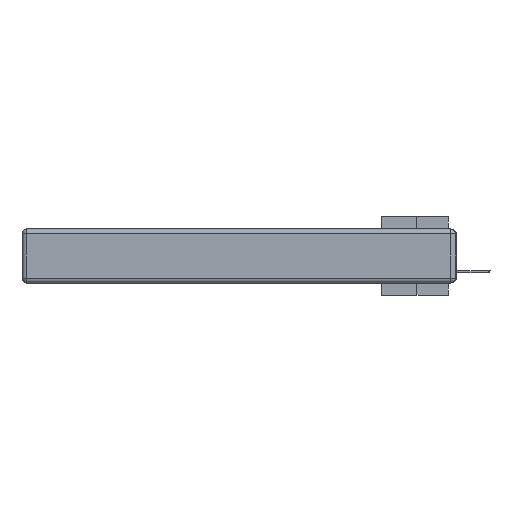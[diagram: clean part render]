
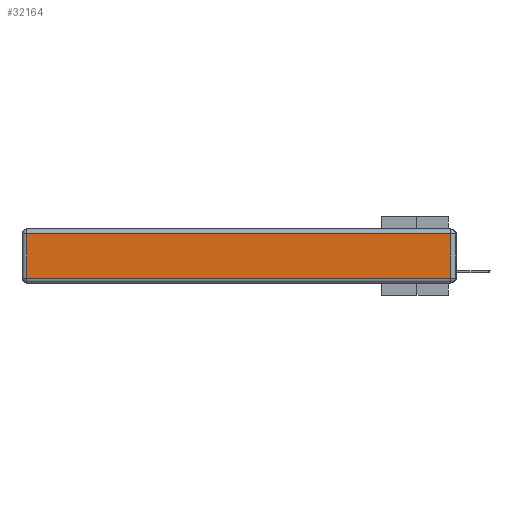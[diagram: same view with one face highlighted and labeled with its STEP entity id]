
A CAD part, left-side view. The second image highlights one B-rep face of the part: STEP entity #32164.
In plain terms, the highlighted planar face has unit normal (-1, 0, 0).
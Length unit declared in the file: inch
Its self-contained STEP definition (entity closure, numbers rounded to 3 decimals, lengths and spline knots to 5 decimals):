
#1705 = ORIENTED_EDGE ( 'NONE', *, *, #19413, .T. ) ;
#3553 = VECTOR ( 'NONE', #9380, 39.37008 ) ;
#4396 = VERTEX_POINT ( 'NONE', #17899 ) ;
#5908 = EDGE_LOOP ( 'NONE', ( #1705, #12740, #26076, #20247 ) ) ;
#6373 = CARTESIAN_POINT ( 'NONE',  ( 0., 0., -0.343 ) ) ;
#6792 = VERTEX_POINT ( 'NONE', #34179 ) ;
#7459 = DIRECTION ( 'NONE',  ( 0., -1., 0. ) ) ;
#8401 = VECTOR ( 'NONE', #7459, 39.37008 ) ;
#8530 = VECTOR ( 'NONE', #11083, 39.37008 ) ;
#9243 = DIRECTION ( 'NONE',  ( -1., 0., 0. ) ) ;
#9380 = DIRECTION ( 'NONE',  ( 0., 1., 0. ) ) ;
#9867 = LINE ( 'NONE', #18057, #3553 ) ;
#10703 = FACE_OUTER_BOUND ( 'NONE', #5908, .T. ) ;
#10829 = CARTESIAN_POINT ( 'NONE',  ( 0., 2.72, -0.343 ) ) ;
#11083 = DIRECTION ( 'NONE',  ( 0., 0., -1. ) ) ;
#11346 = VERTEX_POINT ( 'NONE', #35079 ) ;
#12740 = ORIENTED_EDGE ( 'NONE', *, *, #19407, .T. ) ;
#15490 = DIRECTION ( 'NONE',  ( 0., 0., 1. ) ) ;
#16065 = EDGE_CURVE ( 'NONE', #26657, #6792, #9867, .T. ) ;
#16197 = LINE ( 'NONE', #10829, #8530 ) ;
#17899 = CARTESIAN_POINT ( 'NONE',  ( 0., 0.03, -0.313 ) ) ;
#18057 = CARTESIAN_POINT ( 'NONE',  ( 0., 2.75, -0.03 ) ) ;
#18774 = LINE ( 'NONE', #21575, #8401 ) ;
#19407 = EDGE_CURVE ( 'NONE', #4396, #26657, #21474, .T. ) ;
#19413 = EDGE_CURVE ( 'NONE', #11346, #4396, #18774, .T. ) ;
#20247 = ORIENTED_EDGE ( 'NONE', *, *, #24782, .T. ) ;
#21474 = LINE ( 'NONE', #30043, #30429 ) ;
#21575 = CARTESIAN_POINT ( 'NONE',  ( 0., 0., -0.313 ) ) ;
#24782 = EDGE_CURVE ( 'NONE', #6792, #11346, #16197, .T. ) ;
#26076 = ORIENTED_EDGE ( 'NONE', *, *, #16065, .T. ) ;
#26657 = VERTEX_POINT ( 'NONE', #31685 ) ;
#28320 = AXIS2_PLACEMENT_3D ( 'NONE', #6373, #9243, #35801 ) ;
#30043 = CARTESIAN_POINT ( 'NONE',  ( 0., 0.03, -0.343 ) ) ;
#30429 = VECTOR ( 'NONE', #15490, 39.37008 ) ;
#31685 = CARTESIAN_POINT ( 'NONE',  ( 0., 0.03, -0.03 ) ) ;
#32164 = ADVANCED_FACE ( 'NONE', ( #10703 ), #35938, .T. ) ;
#34179 = CARTESIAN_POINT ( 'NONE',  ( 0., 2.72, -0.03 ) ) ;
#35079 = CARTESIAN_POINT ( 'NONE',  ( 0., 2.72, -0.313 ) ) ;
#35801 = DIRECTION ( 'NONE',  ( 0., 0., 1. ) ) ;
#35938 = PLANE ( 'NONE',  #28320 ) ;
